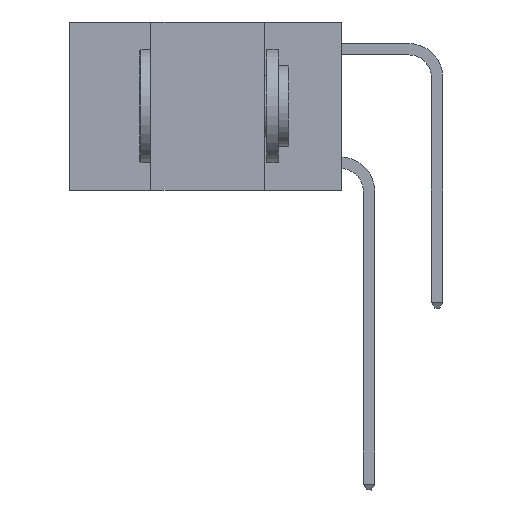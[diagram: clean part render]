
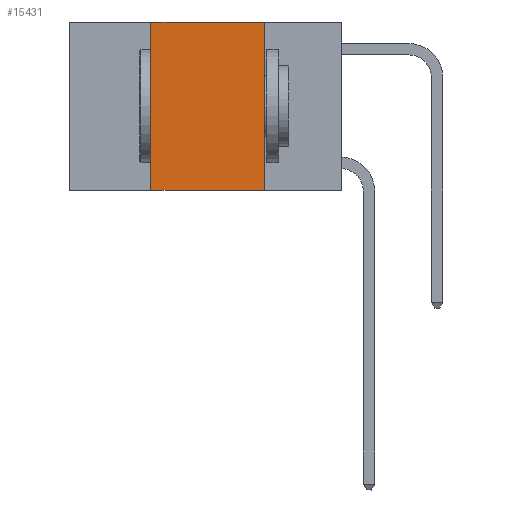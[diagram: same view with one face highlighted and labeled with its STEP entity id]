
A CAD part, left-side view. The second image highlights one B-rep face of the part: STEP entity #15431.
In plain terms, the highlighted planar face has unit normal (-1, 0, 0).
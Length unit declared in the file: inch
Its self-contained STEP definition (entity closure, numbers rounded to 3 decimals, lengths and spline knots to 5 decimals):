
#798 = CARTESIAN_POINT ( 'NONE',  ( 0., 0.6, 0. ) ) ;
#3118 = LINE ( 'NONE', #28582, #6773 ) ;
#5862 = VECTOR ( 'NONE', #17137, 39.37008 ) ;
#6773 = VECTOR ( 'NONE', #24301, 39.37008 ) ;
#7518 = CARTESIAN_POINT ( 'NONE',  ( 0., 0.17, -0.37 ) ) ;
#7620 = EDGE_CURVE ( 'NONE', #20029, #9689, #3118, .T. ) ;
#7911 = DIRECTION ( 'NONE',  ( 0., 0., -1. ) ) ;
#8752 = CARTESIAN_POINT ( 'NONE',  ( 0., 0.6, -0.37 ) ) ;
#9244 = EDGE_CURVE ( 'NONE', #9689, #27072, #10361, .T. ) ;
#9626 = VERTEX_POINT ( 'NONE', #25775 ) ;
#9689 = VERTEX_POINT ( 'NONE', #14866 ) ;
#9882 = DIRECTION ( 'NONE',  ( 1., 0., 0. ) ) ;
#10041 = CARTESIAN_POINT ( 'NONE',  ( 0., 0.42, 0. ) ) ;
#10361 = LINE ( 'NONE', #28994, #28063 ) ;
#11177 = DIRECTION ( 'NONE',  ( 0., -1., 0. ) ) ;
#13642 = ORIENTED_EDGE ( 'NONE', *, *, #23559, .F. ) ;
#14420 = LINE ( 'NONE', #19234, #5862 ) ;
#14866 = CARTESIAN_POINT ( 'NONE',  ( 0., 0.17, 0. ) ) ;
#15431 = ADVANCED_FACE ( 'NONE', ( #23503 ), #26085, .F. ) ;
#16209 = EDGE_CURVE ( 'NONE', #9626, #27072, #22677, .T. ) ;
#17137 = DIRECTION ( 'NONE',  ( 0., 0., 1. ) ) ;
#17177 = VECTOR ( 'NONE', #11177, 39.37008 ) ;
#17462 = DIRECTION ( 'NONE',  ( 0., 0., -1. ) ) ;
#19234 = CARTESIAN_POINT ( 'NONE',  ( 0., 0.42, 0. ) ) ;
#19642 = ORIENTED_EDGE ( 'NONE', *, *, #9244, .F. ) ;
#20029 = VERTEX_POINT ( 'NONE', #10041 ) ;
#20989 = AXIS2_PLACEMENT_3D ( 'NONE', #798, #9882, #7911 ) ;
#22677 = LINE ( 'NONE', #8752, #17177 ) ;
#23503 = FACE_OUTER_BOUND ( 'NONE', #25216, .T. ) ;
#23559 = EDGE_CURVE ( 'NONE', #9626, #20029, #14420, .T. ) ;
#24301 = DIRECTION ( 'NONE',  ( 0., -1., 0. ) ) ;
#25117 = ORIENTED_EDGE ( 'NONE', *, *, #7620, .F. ) ;
#25216 = EDGE_LOOP ( 'NONE', ( #19642, #25117, #13642, #28471 ) ) ;
#25775 = CARTESIAN_POINT ( 'NONE',  ( 0., 0.42, -0.37 ) ) ;
#26085 = PLANE ( 'NONE',  #20989 ) ;
#27072 = VERTEX_POINT ( 'NONE', #7518 ) ;
#28063 = VECTOR ( 'NONE', #17462, 39.37008 ) ;
#28471 = ORIENTED_EDGE ( 'NONE', *, *, #16209, .T. ) ;
#28582 = CARTESIAN_POINT ( 'NONE',  ( 0., 0.6, 0. ) ) ;
#28994 = CARTESIAN_POINT ( 'NONE',  ( 0., 0.17, 0. ) ) ;
